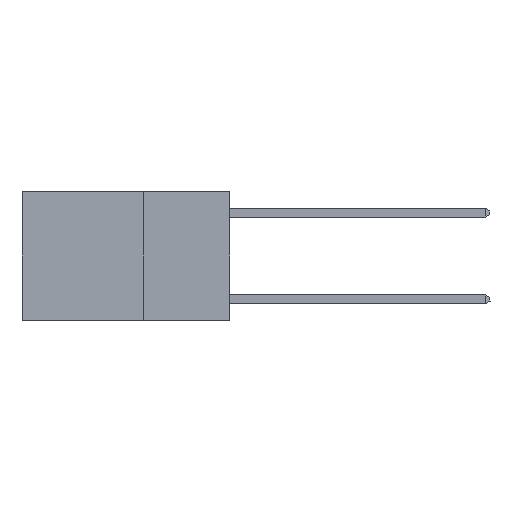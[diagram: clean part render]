
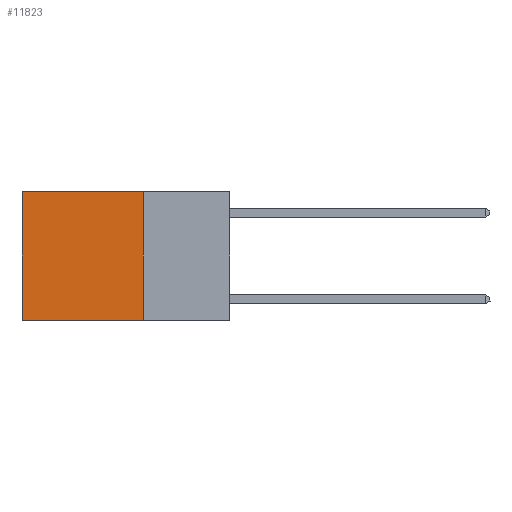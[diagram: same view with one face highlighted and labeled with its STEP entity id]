
A CAD part, left-side view. The second image highlights one B-rep face of the part: STEP entity #11823.
In plain terms, the highlighted planar face has unit normal (-1, 0, 0).
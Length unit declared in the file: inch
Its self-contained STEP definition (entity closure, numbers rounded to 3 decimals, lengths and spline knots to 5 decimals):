
#310 = LINE ( 'NONE', #17210, #1821 ) ;
#1206 = VERTEX_POINT ( 'NONE', #16264 ) ;
#1294 = EDGE_CURVE ( 'NONE', #13584, #1206, #8066, .T. ) ;
#1637 = ORIENTED_EDGE ( 'NONE', *, *, #1294, .T. ) ;
#1821 = VECTOR ( 'NONE', #5891, 39.37008 ) ;
#2211 = CARTESIAN_POINT ( 'NONE',  ( 0.2625, 0.25, 0. ) ) ;
#2291 = DIRECTION ( 'NONE',  ( 0., 1., 0. ) ) ;
#2447 = VERTEX_POINT ( 'NONE', #7449 ) ;
#2452 = VECTOR ( 'NONE', #5401, 39.37008 ) ;
#3451 = VECTOR ( 'NONE', #15032, 39.37008 ) ;
#4034 = CARTESIAN_POINT ( 'NONE',  ( 0.2625, 0.25, 0. ) ) ;
#4589 = ORIENTED_EDGE ( 'NONE', *, *, #14831, .T. ) ;
#4691 = VERTEX_POINT ( 'NONE', #14405 ) ;
#5324 = CARTESIAN_POINT ( 'NONE',  ( 0.2625, 0.25, -0.37 ) ) ;
#5354 = EDGE_CURVE ( 'NONE', #2447, #4691, #6891, .T. ) ;
#5401 = DIRECTION ( 'NONE',  ( 0., 0., -1. ) ) ;
#5891 = DIRECTION ( 'NONE',  ( 0., 0., -1. ) ) ;
#6312 = ORIENTED_EDGE ( 'NONE', *, *, #10354, .F. ) ;
#6891 = LINE ( 'NONE', #5324, #3451 ) ;
#6977 = EDGE_LOOP ( 'NONE', ( #4589, #7754, #6312, #1637 ) ) ;
#7372 = AXIS2_PLACEMENT_3D ( 'NONE', #4034, #13514, #16342 ) ;
#7449 = CARTESIAN_POINT ( 'NONE',  ( 0.2625, 0.25, -0.37 ) ) ;
#7754 = ORIENTED_EDGE ( 'NONE', *, *, #5354, .F. ) ;
#8066 = LINE ( 'NONE', #16352, #11235 ) ;
#10354 = EDGE_CURVE ( 'NONE', #13584, #2447, #13625, .T. ) ;
#11235 = VECTOR ( 'NONE', #2291, 39.37008 ) ;
#11823 = ADVANCED_FACE ( 'NONE', ( #17794 ), #13882, .F. ) ;
#13514 = DIRECTION ( 'NONE',  ( 1., 0., 0. ) ) ;
#13584 = VERTEX_POINT ( 'NONE', #15929 ) ;
#13625 = LINE ( 'NONE', #2211, #2452 ) ;
#13882 = PLANE ( 'NONE',  #7372 ) ;
#14405 = CARTESIAN_POINT ( 'NONE',  ( 0.2625, 0.6, -0.37 ) ) ;
#14831 = EDGE_CURVE ( 'NONE', #1206, #4691, #310, .T. ) ;
#15032 = DIRECTION ( 'NONE',  ( 0., 1., 0. ) ) ;
#15929 = CARTESIAN_POINT ( 'NONE',  ( 0.2625, 0.25, 0. ) ) ;
#16264 = CARTESIAN_POINT ( 'NONE',  ( 0.2625, 0.6, 0. ) ) ;
#16342 = DIRECTION ( 'NONE',  ( 0., 0., -1. ) ) ;
#16352 = CARTESIAN_POINT ( 'NONE',  ( 0.2625, 0.25, 0. ) ) ;
#17210 = CARTESIAN_POINT ( 'NONE',  ( 0.2625, 0.6, 0. ) ) ;
#17794 = FACE_OUTER_BOUND ( 'NONE', #6977, .T. ) ;
